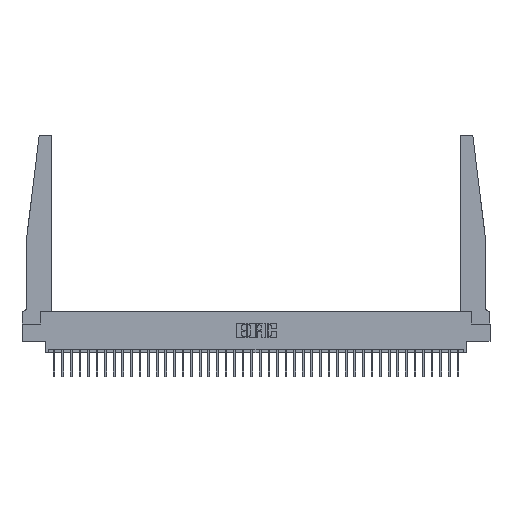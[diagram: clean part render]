
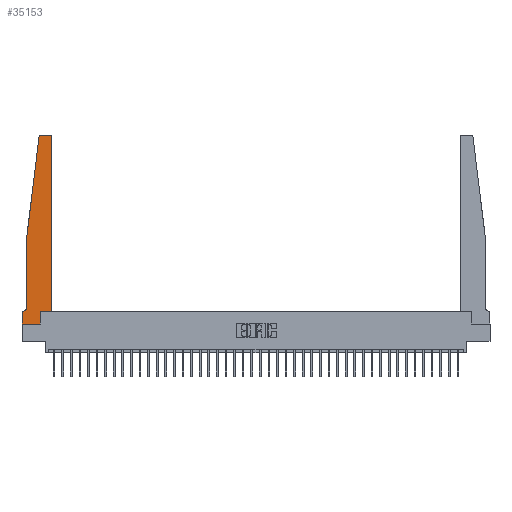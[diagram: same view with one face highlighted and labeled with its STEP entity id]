
A CAD part, top view. The second image highlights one B-rep face of the part: STEP entity #35153.
In plain terms, the highlighted planar face has unit normal (0, 0, 1).
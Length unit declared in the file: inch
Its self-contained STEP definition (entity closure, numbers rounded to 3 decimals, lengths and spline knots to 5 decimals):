
#158 = DIRECTION ( 'NONE',  ( -1., 0., 0. ) ) ;
#1480 = EDGE_CURVE ( 'NONE', #14019, #6793, #26622, .T. ) ;
#1618 = VECTOR ( 'NONE', #20073, 39.37008 ) ;
#1920 = DIRECTION ( 'NONE',  ( -1., 0., 0. ) ) ;
#2135 = ORIENTED_EDGE ( 'NONE', *, *, #26323, .T. ) ;
#2540 = DIRECTION ( 'NONE',  ( 0., 0., -1. ) ) ;
#2623 = LINE ( 'NONE', #28187, #9088 ) ;
#2662 = LINE ( 'NONE', #14967, #16446 ) ;
#2699 = CIRCLE ( 'NONE', #15379, 0.03 ) ;
#2768 = LINE ( 'NONE', #29343, #10085 ) ;
#2781 = CARTESIAN_POINT ( 'NONE',  ( 0.425, 0.18, 0.37 ) ) ;
#2807 = CARTESIAN_POINT ( 'NONE',  ( 0.065, 1.25, 0.37 ) ) ;
#3074 = CARTESIAN_POINT ( 'NONE',  ( 0.27653, 2.75, 0.37 ) ) ;
#3340 = FACE_OUTER_BOUND ( 'NONE', #9640, .T. ) ;
#3785 = CARTESIAN_POINT ( 'NONE',  ( 0.27653, 2.72, 0.37 ) ) ;
#4363 = ORIENTED_EDGE ( 'NONE', *, *, #11620, .T. ) ;
#4598 = VERTEX_POINT ( 'NONE', #12249 ) ;
#5118 = VERTEX_POINT ( 'NONE', #23713 ) ;
#5736 = CARTESIAN_POINT ( 'NONE',  ( 0., 0.1875, 0.37 ) ) ;
#6544 = DIRECTION ( 'NONE',  ( 1., 0., 0. ) ) ;
#6793 = VERTEX_POINT ( 'NONE', #2807 ) ;
#7105 = CARTESIAN_POINT ( 'NONE',  ( 0., 0.1875, 0.37 ) ) ;
#7270 = EDGE_CURVE ( 'NONE', #19649, #25002, #23878, .T. ) ;
#7564 = DIRECTION ( 'NONE',  ( 0., -1., 0. ) ) ;
#7765 = CARTESIAN_POINT ( 'NONE',  ( 0., 0., 0.37 ) ) ;
#7985 = VECTOR ( 'NONE', #158, 39.37008 ) ;
#8513 = DIRECTION ( 'NONE',  ( 1., 0., 0. ) ) ;
#8669 = CARTESIAN_POINT ( 'NONE',  ( 0.065, 1.25, 0.37 ) ) ;
#8751 = LINE ( 'NONE', #12928, #15188 ) ;
#8943 = VERTEX_POINT ( 'NONE', #2781 ) ;
#9067 = ORIENTED_EDGE ( 'NONE', *, *, #12088, .T. ) ;
#9088 = VECTOR ( 'NONE', #30917, 39.37008 ) ;
#9355 = VERTEX_POINT ( 'NONE', #23555 ) ;
#9640 = EDGE_LOOP ( 'NONE', ( #23227, #2135, #31308, #11189, #18524, #34695, #14644, #15511, #9067, #18112, #25375, #4363 ) ) ;
#9683 = LINE ( 'NONE', #27550, #7985 ) ;
#10085 = VECTOR ( 'NONE', #7564, 39.37008 ) ;
#11189 = ORIENTED_EDGE ( 'NONE', *, *, #30900, .T. ) ;
#11620 = EDGE_CURVE ( 'NONE', #9355, #4598, #2699, .T. ) ;
#12088 = EDGE_CURVE ( 'NONE', #5118, #27669, #2662, .T. ) ;
#12249 = CARTESIAN_POINT ( 'NONE',  ( 0.395, 2.75, 0.37 ) ) ;
#12928 = CARTESIAN_POINT ( 'NONE',  ( 0., 0., 0.37 ) ) ;
#13093 = AXIS2_PLACEMENT_3D ( 'NONE', #3785, #22994, #6544 ) ;
#14019 = VERTEX_POINT ( 'NONE', #34175 ) ;
#14644 = ORIENTED_EDGE ( 'NONE', *, *, #21328, .T. ) ;
#14967 = CARTESIAN_POINT ( 'NONE',  ( 0.2605, 0.18, 0.37 ) ) ;
#15188 = VECTOR ( 'NONE', #29321, 39.37008 ) ;
#15379 = AXIS2_PLACEMENT_3D ( 'NONE', #32409, #16084, #35131 ) ;
#15511 = ORIENTED_EDGE ( 'NONE', *, *, #24763, .T. ) ;
#15662 = CARTESIAN_POINT ( 'NONE',  ( 0.065, 0.1875, 0.37 ) ) ;
#15786 = VERTEX_POINT ( 'NONE', #28497 ) ;
#16084 = DIRECTION ( 'NONE',  ( 0., 0., 1. ) ) ;
#16288 = LINE ( 'NONE', #20194, #1618 ) ;
#16309 = DIRECTION ( 'NONE',  ( 0., 1., 0. ) ) ;
#16446 = VECTOR ( 'NONE', #25990, 39.37008 ) ;
#16714 = DIRECTION ( 'NONE',  ( -0.122, -0.992, 0. ) ) ;
#17349 = LINE ( 'NONE', #24569, #23770 ) ;
#18112 = ORIENTED_EDGE ( 'NONE', *, *, #34732, .T. ) ;
#18390 = AXIS2_PLACEMENT_3D ( 'NONE', #19041, #2540, #21788 ) ;
#18520 = VECTOR ( 'NONE', #16714, 39.37008 ) ;
#18524 = ORIENTED_EDGE ( 'NONE', *, *, #24502, .T. ) ;
#19041 = CARTESIAN_POINT ( 'NONE',  ( 0.015, 0.2375, 0.37 ) ) ;
#19469 = CIRCLE ( 'NONE', #18390, 0.05 ) ;
#19649 = VERTEX_POINT ( 'NONE', #28986 ) ;
#19966 = EDGE_CURVE ( 'NONE', #4598, #31192, #9683, .T. ) ;
#20073 = DIRECTION ( 'NONE',  ( 1., 0., 0. ) ) ;
#20194 = CARTESIAN_POINT ( 'NONE',  ( 0.425, 0.18, 0.37 ) ) ;
#21328 = EDGE_CURVE ( 'NONE', #25002, #26013, #8751, .T. ) ;
#21788 = DIRECTION ( 'NONE',  ( -1., 0., 0. ) ) ;
#22202 = PLANE ( 'NONE',  #29556 ) ;
#22994 = DIRECTION ( 'NONE',  ( 0., 0., 1. ) ) ;
#23227 = ORIENTED_EDGE ( 'NONE', *, *, #19966, .T. ) ;
#23555 = CARTESIAN_POINT ( 'NONE',  ( 0.425, 2.72, 0.37 ) ) ;
#23713 = CARTESIAN_POINT ( 'NONE',  ( 0.2605, 0., 0.37 ) ) ;
#23770 = VECTOR ( 'NONE', #16309, 39.37008 ) ;
#23835 = EDGE_CURVE ( 'NONE', #8943, #9355, #17349, .T. ) ;
#23878 = LINE ( 'NONE', #15662, #29385 ) ;
#24502 = EDGE_CURVE ( 'NONE', #15786, #19649, #19469, .T. ) ;
#24569 = CARTESIAN_POINT ( 'NONE',  ( 0.425, 0.18, 0.37 ) ) ;
#24763 = EDGE_CURVE ( 'NONE', #26013, #5118, #2623, .T. ) ;
#24921 = DIRECTION ( 'NONE',  ( 0., 0., 1. ) ) ;
#25002 = VERTEX_POINT ( 'NONE', #7105 ) ;
#25375 = ORIENTED_EDGE ( 'NONE', *, *, #23835, .T. ) ;
#25990 = DIRECTION ( 'NONE',  ( 0., 1., 0. ) ) ;
#26013 = VERTEX_POINT ( 'NONE', #7765 ) ;
#26323 = EDGE_CURVE ( 'NONE', #31192, #14019, #28745, .T. ) ;
#26622 = LINE ( 'NONE', #8669, #18520 ) ;
#27302 = CARTESIAN_POINT ( 'NONE',  ( 0.2605, 0.18, 0.37 ) ) ;
#27550 = CARTESIAN_POINT ( 'NONE',  ( 0.25, 2.75, 0.37 ) ) ;
#27669 = VERTEX_POINT ( 'NONE', #27302 ) ;
#28187 = CARTESIAN_POINT ( 'NONE',  ( 0., 0., 0.37 ) ) ;
#28497 = CARTESIAN_POINT ( 'NONE',  ( 0.065, 0.2375, 0.37 ) ) ;
#28745 = CIRCLE ( 'NONE', #13093, 0.03 ) ;
#28986 = CARTESIAN_POINT ( 'NONE',  ( 0.015, 0.1875, 0.37 ) ) ;
#29321 = DIRECTION ( 'NONE',  ( 0., -1., 0. ) ) ;
#29343 = CARTESIAN_POINT ( 'NONE',  ( 0.065, 1.25, 0.37 ) ) ;
#29385 = VECTOR ( 'NONE', #1920, 39.37008 ) ;
#29556 = AXIS2_PLACEMENT_3D ( 'NONE', #5736, #24921, #8513 ) ;
#30900 = EDGE_CURVE ( 'NONE', #6793, #15786, #2768, .T. ) ;
#30917 = DIRECTION ( 'NONE',  ( 1., 0., 0. ) ) ;
#31192 = VERTEX_POINT ( 'NONE', #3074 ) ;
#31308 = ORIENTED_EDGE ( 'NONE', *, *, #1480, .T. ) ;
#32409 = CARTESIAN_POINT ( 'NONE',  ( 0.395, 2.72, 0.37 ) ) ;
#34175 = CARTESIAN_POINT ( 'NONE',  ( 0.24675, 2.72367, 0.37 ) ) ;
#34695 = ORIENTED_EDGE ( 'NONE', *, *, #7270, .T. ) ;
#34732 = EDGE_CURVE ( 'NONE', #27669, #8943, #16288, .T. ) ;
#35131 = DIRECTION ( 'NONE',  ( 1., 0., 0. ) ) ;
#35153 = ADVANCED_FACE ( 'NONE', ( #3340 ), #22202, .T. ) ;
